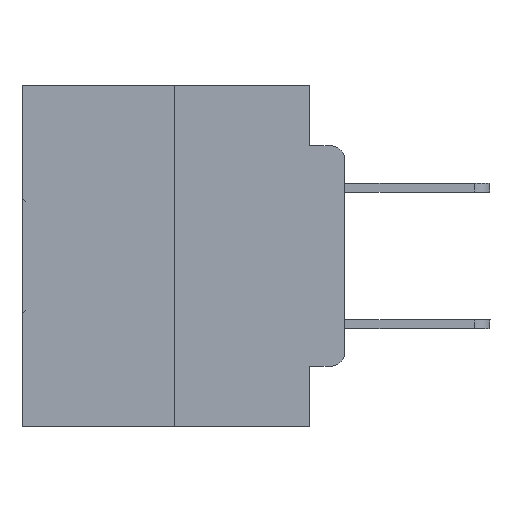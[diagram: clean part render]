
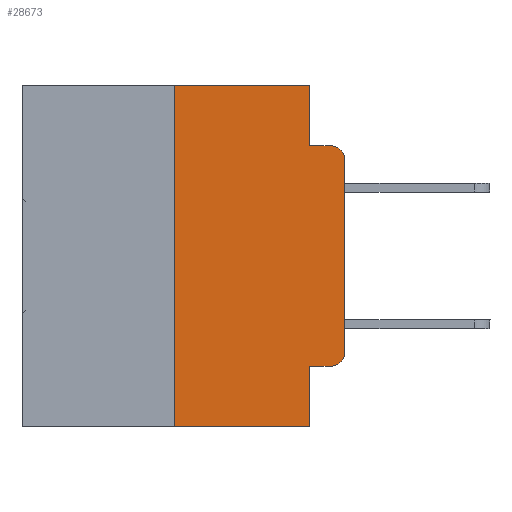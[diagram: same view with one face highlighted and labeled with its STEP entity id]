
A CAD part, left-side view. The second image highlights one B-rep face of the part: STEP entity #28673.
In plain terms, the highlighted planar face has unit normal (-1, 0, 0).
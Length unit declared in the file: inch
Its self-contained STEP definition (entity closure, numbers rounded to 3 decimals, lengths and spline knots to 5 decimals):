
#346 = VERTEX_POINT ( 'NONE', #5636 ) ;
#378 = EDGE_CURVE ( 'NONE', #20888, #6497, #14672, .T. ) ;
#1154 = CARTESIAN_POINT ( 'NONE',  ( 0., 0.051, -0.0885 ) ) ;
#1794 = CARTESIAN_POINT ( 'NONE',  ( 0., 0.02, -0.1085 ) ) ;
#2549 = VECTOR ( 'NONE', #18324, 39.37008 ) ;
#3020 = VECTOR ( 'NONE', #19086, 39.37008 ) ;
#3505 = ORIENTED_EDGE ( 'NONE', *, *, #378, .F. ) ;
#3640 = CARTESIAN_POINT ( 'NONE',  ( 0., 0.051, 0. ) ) ;
#3796 = LINE ( 'NONE', #25525, #22608 ) ;
#4099 = DIRECTION ( 'NONE',  ( 0., -1., 0. ) ) ;
#4375 = CARTESIAN_POINT ( 'NONE',  ( 0., 0.02, -0.3915 ) ) ;
#5406 = CARTESIAN_POINT ( 'NONE',  ( 0., 0.25, -0.5 ) ) ;
#5572 = CARTESIAN_POINT ( 'NONE',  ( 0., 0., -0.3915 ) ) ;
#5636 = CARTESIAN_POINT ( 'NONE',  ( 0., 0.02, -0.0885 ) ) ;
#6497 = VERTEX_POINT ( 'NONE', #3640 ) ;
#6609 = DIRECTION ( 'NONE',  ( 0., 0., -1. ) ) ;
#7467 = VECTOR ( 'NONE', #8812, 39.37008 ) ;
#7545 = ORIENTED_EDGE ( 'NONE', *, *, #11493, .F. ) ;
#7901 = DIRECTION ( 'NONE',  ( 0., 0., 1. ) ) ;
#8398 = DIRECTION ( 'NONE',  ( 0., -1., 0. ) ) ;
#8647 = VERTEX_POINT ( 'NONE', #15685 ) ;
#8812 = DIRECTION ( 'NONE',  ( 0., 0., 1. ) ) ;
#9625 = LINE ( 'NONE', #1154, #13788 ) ;
#9790 = LINE ( 'NONE', #16865, #3020 ) ;
#9833 = CARTESIAN_POINT ( 'NONE',  ( 0., 0.051, -0.0885 ) ) ;
#9933 = VECTOR ( 'NONE', #7901, 39.37008 ) ;
#10093 = ORIENTED_EDGE ( 'NONE', *, *, #17735, .F. ) ;
#10775 = AXIS2_PLACEMENT_3D ( 'NONE', #4375, #23640, #28583 ) ;
#11171 = PLANE ( 'NONE',  #29701 ) ;
#11272 = CARTESIAN_POINT ( 'NONE',  ( 0., 0.473, 0. ) ) ;
#11493 = EDGE_CURVE ( 'NONE', #22517, #20888, #30287, .T. ) ;
#11712 = VERTEX_POINT ( 'NONE', #5572 ) ;
#12504 = EDGE_CURVE ( 'NONE', #8647, #346, #26401, .T. ) ;
#12933 = ORIENTED_EDGE ( 'NONE', *, *, #14191, .T. ) ;
#13255 = CARTESIAN_POINT ( 'NONE',  ( 0., 0.473, 0. ) ) ;
#13378 = CARTESIAN_POINT ( 'NONE',  ( 0., 0.051, -0.4115 ) ) ;
#13418 = EDGE_CURVE ( 'NONE', #6497, #16033, #9790, .T. ) ;
#13694 = DIRECTION ( 'NONE',  ( 1., 0., 0. ) ) ;
#13788 = VECTOR ( 'NONE', #8398, 39.37008 ) ;
#14191 = EDGE_CURVE ( 'NONE', #11712, #8647, #16521, .T. ) ;
#14416 = EDGE_CURVE ( 'NONE', #21246, #11712, #23656, .T. ) ;
#14672 = LINE ( 'NONE', #13255, #22588 ) ;
#14818 = ORIENTED_EDGE ( 'NONE', *, *, #14416, .T. ) ;
#14979 = CARTESIAN_POINT ( 'NONE',  ( 0., 0.25, 0. ) ) ;
#15685 = CARTESIAN_POINT ( 'NONE',  ( 0., 0., -0.1085 ) ) ;
#15821 = DIRECTION ( 'NONE',  ( -1., 0., 0. ) ) ;
#16033 = VERTEX_POINT ( 'NONE', #9833 ) ;
#16113 = EDGE_CURVE ( 'NONE', #16033, #346, #9625, .T. ) ;
#16521 = LINE ( 'NONE', #18302, #7467 ) ;
#16543 = CARTESIAN_POINT ( 'NONE',  ( 0., 0.051, -0.4115 ) ) ;
#16597 = CARTESIAN_POINT ( 'NONE',  ( 0., 0.02, -0.4115 ) ) ;
#16865 = CARTESIAN_POINT ( 'NONE',  ( 0., 0.051, 0. ) ) ;
#17735 = EDGE_CURVE ( 'NONE', #28139, #21541, #3796, .T. ) ;
#18233 = ORIENTED_EDGE ( 'NONE', *, *, #13418, .F. ) ;
#18302 = CARTESIAN_POINT ( 'NONE',  ( 0., 0., 0. ) ) ;
#18324 = DIRECTION ( 'NONE',  ( 0., -1., 0. ) ) ;
#18992 = DIRECTION ( 'NONE',  ( 0., 0., -1. ) ) ;
#19086 = DIRECTION ( 'NONE',  ( 0., 0., -1. ) ) ;
#19872 = VECTOR ( 'NONE', #4099, 39.37008 ) ;
#20539 = CARTESIAN_POINT ( 'NONE',  ( 0., 0.25, 0. ) ) ;
#20888 = VERTEX_POINT ( 'NONE', #20539 ) ;
#21246 = VERTEX_POINT ( 'NONE', #16597 ) ;
#21541 = VERTEX_POINT ( 'NONE', #22999 ) ;
#22517 = VERTEX_POINT ( 'NONE', #5406 ) ;
#22538 = ORIENTED_EDGE ( 'NONE', *, *, #28614, .T. ) ;
#22588 = VECTOR ( 'NONE', #30016, 39.37008 ) ;
#22608 = VECTOR ( 'NONE', #18992, 39.37008 ) ;
#22999 = CARTESIAN_POINT ( 'NONE',  ( 0., 0.051, -0.5 ) ) ;
#23640 = DIRECTION ( 'NONE',  ( -1., 0., 0. ) ) ;
#23656 = CIRCLE ( 'NONE', #10775, 0.02 ) ;
#25525 = CARTESIAN_POINT ( 'NONE',  ( 0., 0.051, 0. ) ) ;
#25538 = ORIENTED_EDGE ( 'NONE', *, *, #16113, .F. ) ;
#25768 = CARTESIAN_POINT ( 'NONE',  ( 0., 0.473, -0.5 ) ) ;
#26401 = CIRCLE ( 'NONE', #29483, 0.02 ) ;
#27104 = EDGE_LOOP ( 'NONE', ( #12933, #27989, #25538, #18233, #3505, #7545, #28744, #10093, #22538, #14818 ) ) ;
#27755 = LINE ( 'NONE', #25768, #19872 ) ;
#27989 = ORIENTED_EDGE ( 'NONE', *, *, #12504, .T. ) ;
#28139 = VERTEX_POINT ( 'NONE', #16543 ) ;
#28172 = LINE ( 'NONE', #13378, #2549 ) ;
#28533 = FACE_OUTER_BOUND ( 'NONE', #27104, .T. ) ;
#28583 = DIRECTION ( 'NONE',  ( 0., 0., -1. ) ) ;
#28614 = EDGE_CURVE ( 'NONE', #28139, #21246, #28172, .T. ) ;
#28673 = ADVANCED_FACE ( 'NONE', ( #28533 ), #11171, .F. ) ;
#28744 = ORIENTED_EDGE ( 'NONE', *, *, #30636, .T. ) ;
#29483 = AXIS2_PLACEMENT_3D ( 'NONE', #1794, #15821, #6609 ) ;
#29701 = AXIS2_PLACEMENT_3D ( 'NONE', #11272, #13694, #30534 ) ;
#30016 = DIRECTION ( 'NONE',  ( 0., -1., 0. ) ) ;
#30287 = LINE ( 'NONE', #14979, #9933 ) ;
#30534 = DIRECTION ( 'NONE',  ( 0., 0., -1. ) ) ;
#30636 = EDGE_CURVE ( 'NONE', #22517, #21541, #27755, .T. ) ;
